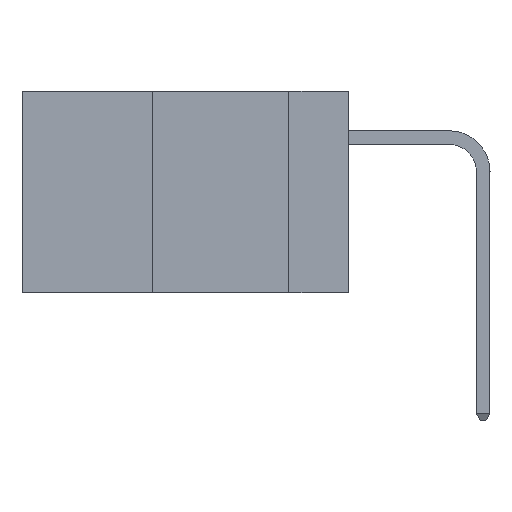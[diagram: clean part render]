
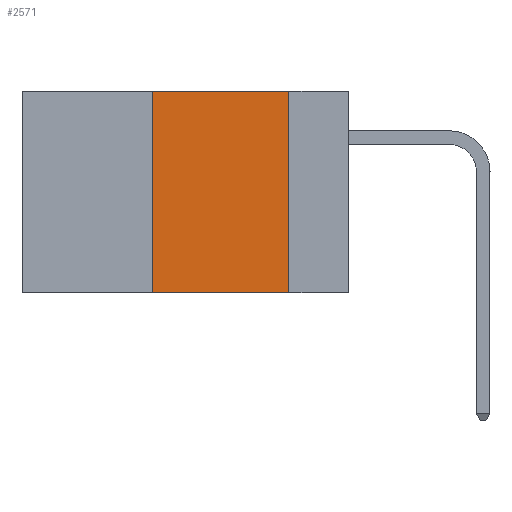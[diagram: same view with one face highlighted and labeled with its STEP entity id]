
A CAD part, left-side view. The second image highlights one B-rep face of the part: STEP entity #2571.
In plain terms, the highlighted planar face has unit normal (-1, 0, 0).
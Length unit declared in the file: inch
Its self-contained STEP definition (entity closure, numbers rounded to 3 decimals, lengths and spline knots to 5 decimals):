
#1 = CARTESIAN_POINT ( 'NONE',  ( 0., 0.36, -0.37 ) ) ;
#611 = VERTEX_POINT ( 'NONE', #1 ) ;
#689 = DIRECTION ( 'NONE',  ( 0., 0., -1. ) ) ;
#1793 = LINE ( 'NONE', #5601, #12936 ) ;
#1798 = CARTESIAN_POINT ( 'NONE',  ( 0., 0.11, 0. ) ) ;
#2571 = ADVANCED_FACE ( 'NONE', ( #9607 ), #13507, .F. ) ;
#2938 = AXIS2_PLACEMENT_3D ( 'NONE', #14698, #3222, #16146 ) ;
#3012 = VECTOR ( 'NONE', #11781, 39.37008 ) ;
#3222 = DIRECTION ( 'NONE',  ( 1., 0., 0. ) ) ;
#3916 = EDGE_CURVE ( 'NONE', #6973, #13711, #1793, .T. ) ;
#3937 = CARTESIAN_POINT ( 'NONE',  ( 0., 0.36, 0. ) ) ;
#4013 = LINE ( 'NONE', #3937, #14679 ) ;
#4264 = CARTESIAN_POINT ( 'NONE',  ( 0., 0.36, 0. ) ) ;
#5601 = CARTESIAN_POINT ( 'NONE',  ( 0., 0.11, 0. ) ) ;
#6008 = LINE ( 'NONE', #6168, #15214 ) ;
#6168 = CARTESIAN_POINT ( 'NONE',  ( 0., 0.6, -0.37 ) ) ;
#6516 = VERTEX_POINT ( 'NONE', #4264 ) ;
#6973 = VERTEX_POINT ( 'NONE', #1798 ) ;
#7753 = EDGE_CURVE ( 'NONE', #6516, #6973, #8189, .T. ) ;
#8189 = LINE ( 'NONE', #9322, #3012 ) ;
#8283 = EDGE_LOOP ( 'NONE', ( #14437, #9671, #14669, #10762 ) ) ;
#8424 = CARTESIAN_POINT ( 'NONE',  ( 0., 0.11, -0.37 ) ) ;
#8955 = DIRECTION ( 'NONE',  ( 0., 0., 1. ) ) ;
#9322 = CARTESIAN_POINT ( 'NONE',  ( 0., 0.6, 0. ) ) ;
#9607 = FACE_OUTER_BOUND ( 'NONE', #8283, .T. ) ;
#9671 = ORIENTED_EDGE ( 'NONE', *, *, #7753, .F. ) ;
#10114 = EDGE_CURVE ( 'NONE', #611, #13711, #6008, .T. ) ;
#10762 = ORIENTED_EDGE ( 'NONE', *, *, #10114, .T. ) ;
#11222 = DIRECTION ( 'NONE',  ( 0., -1., 0. ) ) ;
#11781 = DIRECTION ( 'NONE',  ( 0., -1., 0. ) ) ;
#12936 = VECTOR ( 'NONE', #689, 39.37008 ) ;
#13507 = PLANE ( 'NONE',  #2938 ) ;
#13711 = VERTEX_POINT ( 'NONE', #8424 ) ;
#14437 = ORIENTED_EDGE ( 'NONE', *, *, #3916, .F. ) ;
#14669 = ORIENTED_EDGE ( 'NONE', *, *, #16477, .F. ) ;
#14679 = VECTOR ( 'NONE', #8955, 39.37008 ) ;
#14698 = CARTESIAN_POINT ( 'NONE',  ( 0., 0.6, 0. ) ) ;
#15214 = VECTOR ( 'NONE', #11222, 39.37008 ) ;
#16146 = DIRECTION ( 'NONE',  ( 0., 0., -1. ) ) ;
#16477 = EDGE_CURVE ( 'NONE', #611, #6516, #4013, .T. ) ;
